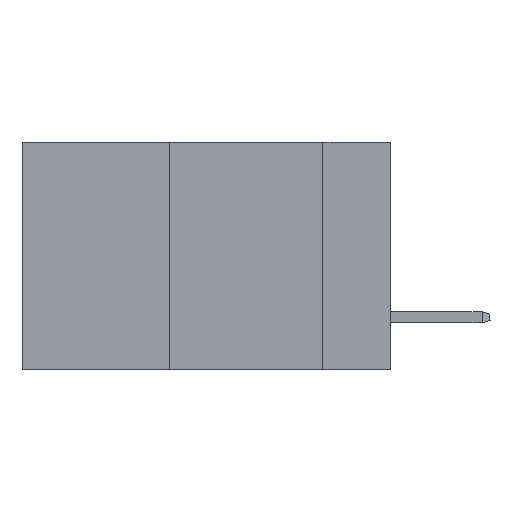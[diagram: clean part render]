
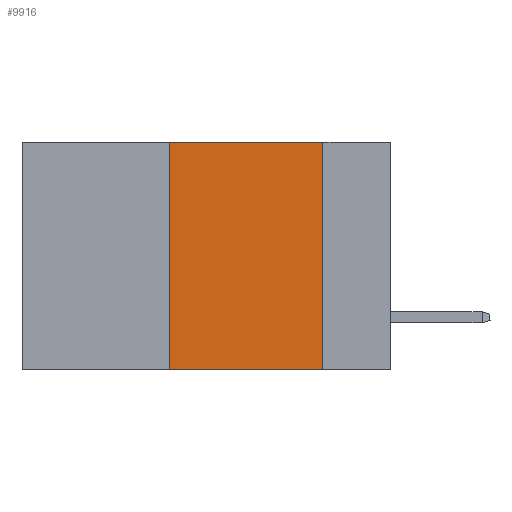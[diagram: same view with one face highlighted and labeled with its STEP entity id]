
A CAD part, left-side view. The second image highlights one B-rep face of the part: STEP entity #9916.
In plain terms, the highlighted planar face has unit normal (-1, 0, 0).
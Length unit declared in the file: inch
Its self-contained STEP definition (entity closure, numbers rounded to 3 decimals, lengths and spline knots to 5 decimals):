
#40 = VERTEX_POINT ( 'NONE', #6170 ) ;
#971 = ORIENTED_EDGE ( 'NONE', *, *, #15218, .T. ) ;
#1173 = LINE ( 'NONE', #4168, #10583 ) ;
#1186 = DIRECTION ( 'NONE',  ( 1., 0., 0. ) ) ;
#1564 = CARTESIAN_POINT ( 'NONE',  ( 0., 0.11, -0.37 ) ) ;
#1661 = ORIENTED_EDGE ( 'NONE', *, *, #10160, .F. ) ;
#2313 = PLANE ( 'NONE',  #12441 ) ;
#2658 = VECTOR ( 'NONE', #12865, 39.37008 ) ;
#3115 = VECTOR ( 'NONE', #7850, 39.37008 ) ;
#3995 = VERTEX_POINT ( 'NONE', #14214 ) ;
#4065 = VERTEX_POINT ( 'NONE', #1564 ) ;
#4168 = CARTESIAN_POINT ( 'NONE',  ( 0., 0.6, -0.37 ) ) ;
#4376 = LINE ( 'NONE', #10989, #14813 ) ;
#5345 = FACE_OUTER_BOUND ( 'NONE', #12411, .T. ) ;
#6170 = CARTESIAN_POINT ( 'NONE',  ( 0., 0.11, 0. ) ) ;
#6791 = ORIENTED_EDGE ( 'NONE', *, *, #11267, .F. ) ;
#6904 = CARTESIAN_POINT ( 'NONE',  ( 0., 0.36, 0. ) ) ;
#7730 = CARTESIAN_POINT ( 'NONE',  ( 0., 0.6, 0. ) ) ;
#7850 = DIRECTION ( 'NONE',  ( 0., 0., -1. ) ) ;
#8233 = EDGE_CURVE ( 'NONE', #40, #4065, #15840, .T. ) ;
#8632 = VERTEX_POINT ( 'NONE', #6904 ) ;
#9821 = DIRECTION ( 'NONE',  ( 0., 0., 1. ) ) ;
#9916 = ADVANCED_FACE ( 'NONE', ( #5345 ), #2313, .F. ) ;
#10160 = EDGE_CURVE ( 'NONE', #8632, #40, #14135, .T. ) ;
#10583 = VECTOR ( 'NONE', #10806, 39.37008 ) ;
#10806 = DIRECTION ( 'NONE',  ( 0., -1., 0. ) ) ;
#10961 = ORIENTED_EDGE ( 'NONE', *, *, #8233, .F. ) ;
#10989 = CARTESIAN_POINT ( 'NONE',  ( 0., 0.36, 0. ) ) ;
#11267 = EDGE_CURVE ( 'NONE', #3995, #8632, #4376, .T. ) ;
#12411 = EDGE_LOOP ( 'NONE', ( #10961, #1661, #6791, #971 ) ) ;
#12441 = AXIS2_PLACEMENT_3D ( 'NONE', #15554, #1186, #13054 ) ;
#12865 = DIRECTION ( 'NONE',  ( 0., -1., 0. ) ) ;
#13054 = DIRECTION ( 'NONE',  ( 0., 0., -1. ) ) ;
#13322 = CARTESIAN_POINT ( 'NONE',  ( 0., 0.11, 0. ) ) ;
#14135 = LINE ( 'NONE', #7730, #2658 ) ;
#14214 = CARTESIAN_POINT ( 'NONE',  ( 0., 0.36, -0.37 ) ) ;
#14813 = VECTOR ( 'NONE', #9821, 39.37008 ) ;
#15218 = EDGE_CURVE ( 'NONE', #3995, #4065, #1173, .T. ) ;
#15554 = CARTESIAN_POINT ( 'NONE',  ( 0., 0.6, 0. ) ) ;
#15840 = LINE ( 'NONE', #13322, #3115 ) ;
